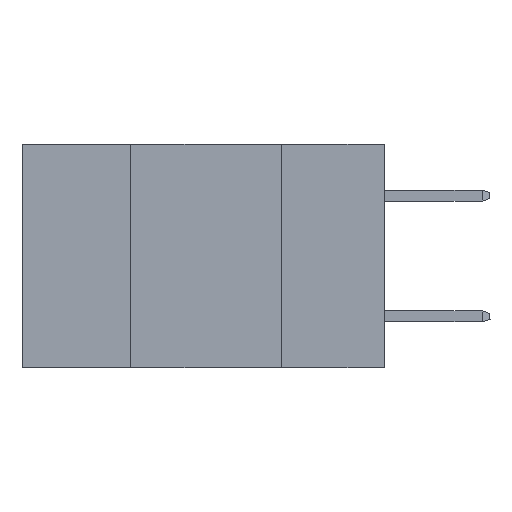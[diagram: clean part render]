
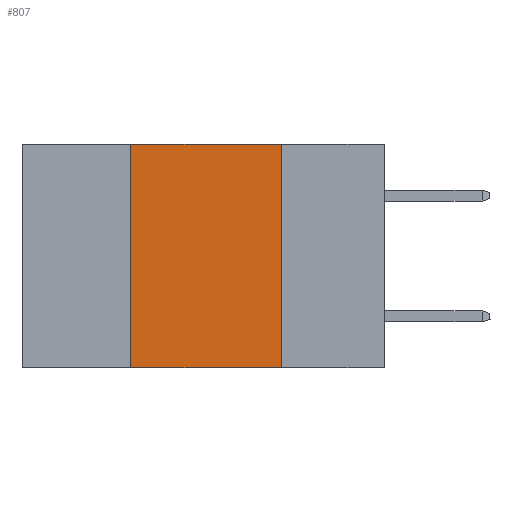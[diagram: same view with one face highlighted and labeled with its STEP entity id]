
A CAD part, left-side view. The second image highlights one B-rep face of the part: STEP entity #807.
In plain terms, the highlighted planar face has unit normal (-1, 0, 0).
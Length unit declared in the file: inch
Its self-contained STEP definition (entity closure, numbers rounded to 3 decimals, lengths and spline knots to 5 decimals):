
#805 = LINE ( 'NONE', #4707, #7187 ) ;
#807 = ADVANCED_FACE ( 'NONE', ( #12481 ), #10455, .F. ) ;
#1961 = CARTESIAN_POINT ( 'NONE',  ( 0., 0.42, 0. ) ) ;
#2188 = AXIS2_PLACEMENT_3D ( 'NONE', #10577, #10469, #10843 ) ;
#2244 = ORIENTED_EDGE ( 'NONE', *, *, #7204, .T. ) ;
#2628 = EDGE_CURVE ( 'NONE', #7787, #13027, #16968, .T. ) ;
#2823 = CARTESIAN_POINT ( 'NONE',  ( 0., 0.17, -0.37 ) ) ;
#2942 = VECTOR ( 'NONE', #3322, 39.37008 ) ;
#3322 = DIRECTION ( 'NONE',  ( 0., 0., -1. ) ) ;
#3619 = DIRECTION ( 'NONE',  ( 0., 0., 1. ) ) ;
#4442 = EDGE_CURVE ( 'NONE', #10096, #7787, #805, .T. ) ;
#4525 = CARTESIAN_POINT ( 'NONE',  ( 0., 0.42, -0.37 ) ) ;
#4604 = DIRECTION ( 'NONE',  ( 0., -1., 0. ) ) ;
#4707 = CARTESIAN_POINT ( 'NONE',  ( 0., 0.6, 0. ) ) ;
#4968 = CARTESIAN_POINT ( 'NONE',  ( 0., 0.17, -0.37 ) ) ;
#6244 = CARTESIAN_POINT ( 'NONE',  ( 0., 0.42, -0.37 ) ) ;
#6283 = EDGE_CURVE ( 'NONE', #8112, #10096, #13820, .T. ) ;
#6992 = EDGE_LOOP ( 'NONE', ( #13553, #15547, #15931, #2244 ) ) ;
#7187 = VECTOR ( 'NONE', #4604, 39.37008 ) ;
#7204 = EDGE_CURVE ( 'NONE', #8112, #13027, #14183, .T. ) ;
#7787 = VERTEX_POINT ( 'NONE', #7990 ) ;
#7990 = CARTESIAN_POINT ( 'NONE',  ( 0., 0.17, 0. ) ) ;
#8112 = VERTEX_POINT ( 'NONE', #6244 ) ;
#10096 = VERTEX_POINT ( 'NONE', #1961 ) ;
#10392 = VECTOR ( 'NONE', #3619, 39.37008 ) ;
#10455 = PLANE ( 'NONE',  #2188 ) ;
#10469 = DIRECTION ( 'NONE',  ( 1., 0., 0. ) ) ;
#10577 = CARTESIAN_POINT ( 'NONE',  ( 0., 0.6, 0. ) ) ;
#10843 = DIRECTION ( 'NONE',  ( 0., 0., -1. ) ) ;
#12481 = FACE_OUTER_BOUND ( 'NONE', #6992, .T. ) ;
#13027 = VERTEX_POINT ( 'NONE', #4968 ) ;
#13495 = CARTESIAN_POINT ( 'NONE',  ( 0., 0.6, -0.37 ) ) ;
#13553 = ORIENTED_EDGE ( 'NONE', *, *, #2628, .F. ) ;
#13820 = LINE ( 'NONE', #4525, #10392 ) ;
#14183 = LINE ( 'NONE', #13495, #17109 ) ;
#15006 = DIRECTION ( 'NONE',  ( 0., -1., 0. ) ) ;
#15547 = ORIENTED_EDGE ( 'NONE', *, *, #4442, .F. ) ;
#15931 = ORIENTED_EDGE ( 'NONE', *, *, #6283, .F. ) ;
#16968 = LINE ( 'NONE', #2823, #2942 ) ;
#17109 = VECTOR ( 'NONE', #15006, 39.37008 ) ;
